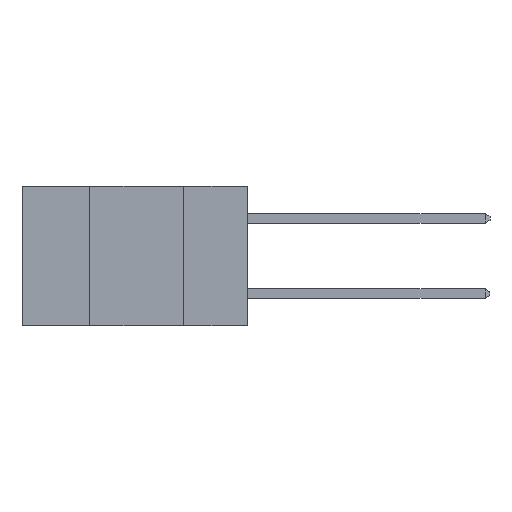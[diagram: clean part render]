
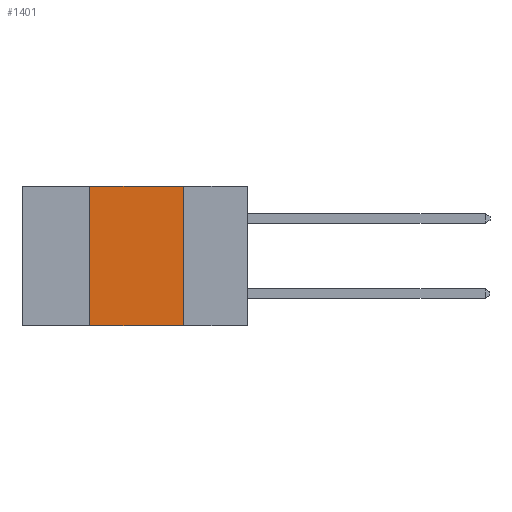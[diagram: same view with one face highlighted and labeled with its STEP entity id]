
A CAD part, left-side view. The second image highlights one B-rep face of the part: STEP entity #1401.
In plain terms, the highlighted planar face has unit normal (-1, 0, 0).
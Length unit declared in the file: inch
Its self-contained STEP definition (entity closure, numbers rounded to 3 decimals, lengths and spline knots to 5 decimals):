
#245 = VECTOR ( 'NONE', #505, 39.37008 ) ;
#463 = CARTESIAN_POINT ( 'NONE',  ( 0., 0.42, -0.37 ) ) ;
#505 = DIRECTION ( 'NONE',  ( 0., 0., -1. ) ) ;
#809 = VECTOR ( 'NONE', #8608, 39.37008 ) ;
#1043 = VECTOR ( 'NONE', #5216, 39.37008 ) ;
#1078 = DIRECTION ( 'NONE',  ( 0., 0., -1. ) ) ;
#1150 = CARTESIAN_POINT ( 'NONE',  ( 0., 0.17, 0. ) ) ;
#1255 = EDGE_CURVE ( 'NONE', #5052, #3864, #2530, .T. ) ;
#1336 = LINE ( 'NONE', #9918, #809 ) ;
#1401 = ADVANCED_FACE ( 'NONE', ( #9271 ), #3317, .F. ) ;
#1422 = VECTOR ( 'NONE', #5278, 39.37008 ) ;
#1805 = EDGE_LOOP ( 'NONE', ( #4160, #5364, #6663, #4182 ) ) ;
#2530 = LINE ( 'NONE', #1150, #245 ) ;
#2617 = CARTESIAN_POINT ( 'NONE',  ( 0., 0.17, 0. ) ) ;
#2785 = VERTEX_POINT ( 'NONE', #463 ) ;
#2820 = AXIS2_PLACEMENT_3D ( 'NONE', #3925, #9960, #1078 ) ;
#3084 = LINE ( 'NONE', #9563, #1043 ) ;
#3176 = LINE ( 'NONE', #5284, #1422 ) ;
#3317 = PLANE ( 'NONE',  #2820 ) ;
#3831 = VERTEX_POINT ( 'NONE', #4909 ) ;
#3864 = VERTEX_POINT ( 'NONE', #5557 ) ;
#3925 = CARTESIAN_POINT ( 'NONE',  ( 0., 0.6, 0. ) ) ;
#4160 = ORIENTED_EDGE ( 'NONE', *, *, #1255, .F. ) ;
#4182 = ORIENTED_EDGE ( 'NONE', *, *, #8437, .T. ) ;
#4909 = CARTESIAN_POINT ( 'NONE',  ( 0., 0.42, 0. ) ) ;
#5052 = VERTEX_POINT ( 'NONE', #2617 ) ;
#5216 = DIRECTION ( 'NONE',  ( 0., 0., 1. ) ) ;
#5278 = DIRECTION ( 'NONE',  ( 0., -1., 0. ) ) ;
#5284 = CARTESIAN_POINT ( 'NONE',  ( 0., 0.6, 0. ) ) ;
#5364 = ORIENTED_EDGE ( 'NONE', *, *, #7205, .F. ) ;
#5557 = CARTESIAN_POINT ( 'NONE',  ( 0., 0.17, -0.37 ) ) ;
#6663 = ORIENTED_EDGE ( 'NONE', *, *, #9773, .F. ) ;
#7205 = EDGE_CURVE ( 'NONE', #3831, #5052, #3176, .T. ) ;
#8437 = EDGE_CURVE ( 'NONE', #2785, #3864, #1336, .T. ) ;
#8608 = DIRECTION ( 'NONE',  ( 0., -1., 0. ) ) ;
#9271 = FACE_OUTER_BOUND ( 'NONE', #1805, .T. ) ;
#9563 = CARTESIAN_POINT ( 'NONE',  ( 0., 0.42, 0. ) ) ;
#9773 = EDGE_CURVE ( 'NONE', #2785, #3831, #3084, .T. ) ;
#9918 = CARTESIAN_POINT ( 'NONE',  ( 0., 0.6, -0.37 ) ) ;
#9960 = DIRECTION ( 'NONE',  ( 1., 0., 0. ) ) ;
